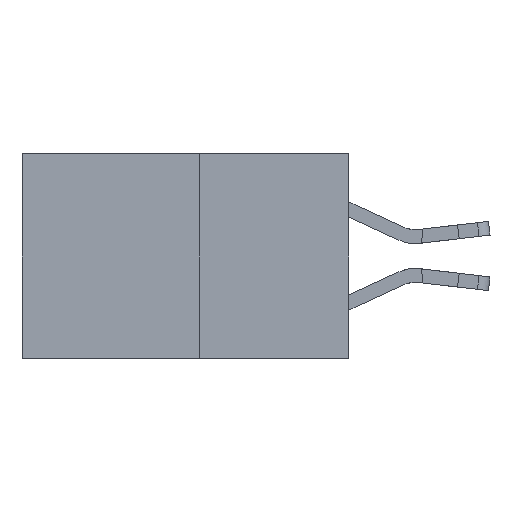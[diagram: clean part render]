
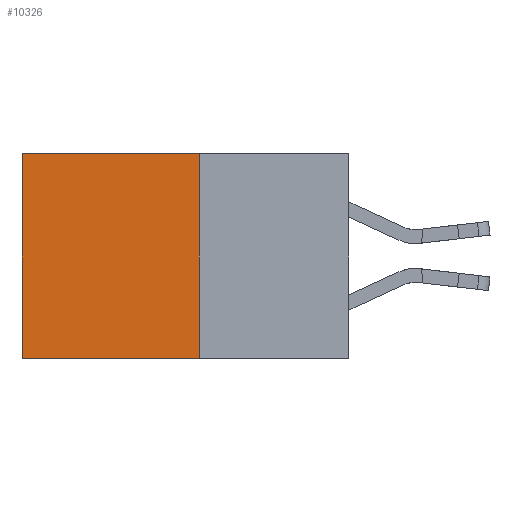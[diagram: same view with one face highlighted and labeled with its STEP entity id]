
A CAD part, left-side view. The second image highlights one B-rep face of the part: STEP entity #10326.
In plain terms, the highlighted planar face has unit normal (-1, 0, 0).
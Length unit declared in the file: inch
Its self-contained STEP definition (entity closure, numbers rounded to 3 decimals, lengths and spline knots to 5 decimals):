
#195 = CARTESIAN_POINT ( 'NONE',  ( 0.277, 0.27, -0.37 ) ) ;
#696 = VECTOR ( 'NONE', #16158, 39.37008 ) ;
#1803 = VERTEX_POINT ( 'NONE', #7052 ) ;
#1915 = LINE ( 'NONE', #13023, #8291 ) ;
#3535 = VERTEX_POINT ( 'NONE', #15232 ) ;
#3795 = ORIENTED_EDGE ( 'NONE', *, *, #12134, .T. ) ;
#4078 = EDGE_CURVE ( 'NONE', #7336, #3535, #15440, .T. ) ;
#4300 = VECTOR ( 'NONE', #6756, 39.37008 ) ;
#4779 = FACE_OUTER_BOUND ( 'NONE', #6221, .T. ) ;
#4892 = LINE ( 'NONE', #14868, #696 ) ;
#5079 = VECTOR ( 'NONE', #14043, 39.37008 ) ;
#6221 = EDGE_LOOP ( 'NONE', ( #8535, #7627, #14196, #3795 ) ) ;
#6508 = DIRECTION ( 'NONE',  ( 0., 0., -1. ) ) ;
#6621 = PLANE ( 'NONE',  #9484 ) ;
#6756 = DIRECTION ( 'NONE',  ( 0., 1., 0. ) ) ;
#7052 = CARTESIAN_POINT ( 'NONE',  ( 0.277, 0.59, 0. ) ) ;
#7336 = VERTEX_POINT ( 'NONE', #195 ) ;
#7627 = ORIENTED_EDGE ( 'NONE', *, *, #4078, .F. ) ;
#7706 = EDGE_CURVE ( 'NONE', #15804, #7336, #1915, .T. ) ;
#8291 = VECTOR ( 'NONE', #6508, 39.37008 ) ;
#8535 = ORIENTED_EDGE ( 'NONE', *, *, #13739, .T. ) ;
#9268 = DIRECTION ( 'NONE',  ( 0., 0., -1. ) ) ;
#9484 = AXIS2_PLACEMENT_3D ( 'NONE', #15630, #16894, #9268 ) ;
#10326 = ADVANCED_FACE ( 'NONE', ( #4779 ), #6621, .F. ) ;
#12134 = EDGE_CURVE ( 'NONE', #15804, #1803, #15102, .T. ) ;
#13023 = CARTESIAN_POINT ( 'NONE',  ( 0.277, 0.27, -0.37 ) ) ;
#13100 = CARTESIAN_POINT ( 'NONE',  ( 0.277, 0.27, -0.37 ) ) ;
#13739 = EDGE_CURVE ( 'NONE', #1803, #3535, #4892, .T. ) ;
#14043 = DIRECTION ( 'NONE',  ( 0., 1., 0. ) ) ;
#14196 = ORIENTED_EDGE ( 'NONE', *, *, #7706, .F. ) ;
#14868 = CARTESIAN_POINT ( 'NONE',  ( 0.277, 0.59, -0.37 ) ) ;
#15102 = LINE ( 'NONE', #17017, #4300 ) ;
#15232 = CARTESIAN_POINT ( 'NONE',  ( 0.277, 0.59, -0.37 ) ) ;
#15292 = CARTESIAN_POINT ( 'NONE',  ( 0.277, 0.27, 0. ) ) ;
#15440 = LINE ( 'NONE', #13100, #5079 ) ;
#15630 = CARTESIAN_POINT ( 'NONE',  ( 0.277, 0.27, -0.37 ) ) ;
#15804 = VERTEX_POINT ( 'NONE', #15292 ) ;
#16158 = DIRECTION ( 'NONE',  ( 0., 0., -1. ) ) ;
#16894 = DIRECTION ( 'NONE',  ( 1., 0., 0. ) ) ;
#17017 = CARTESIAN_POINT ( 'NONE',  ( 0.277, 0.27, 0. ) ) ;
